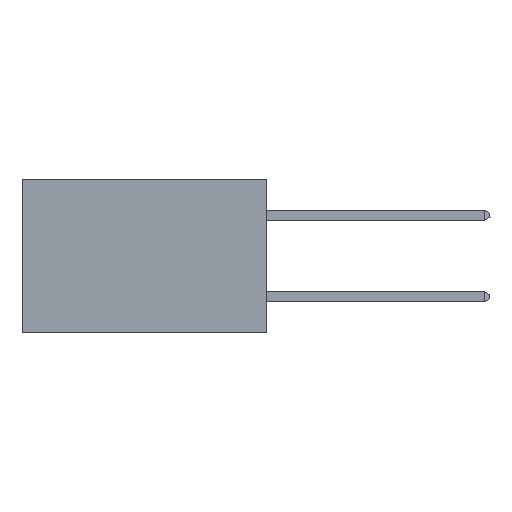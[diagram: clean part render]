
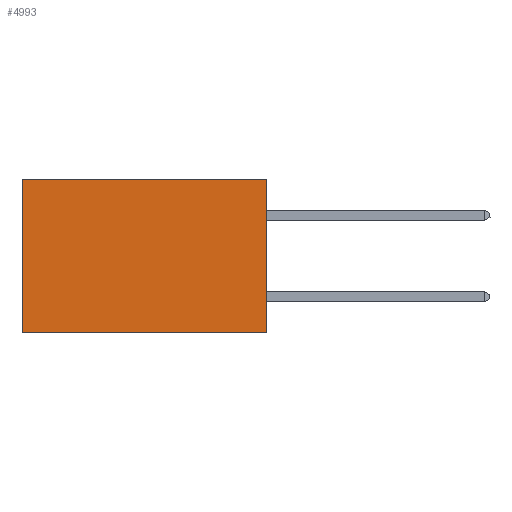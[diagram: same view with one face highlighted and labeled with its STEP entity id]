
A CAD part, left-side view. The second image highlights one B-rep face of the part: STEP entity #4993.
In plain terms, the highlighted planar face has unit normal (-1, 0, 0).
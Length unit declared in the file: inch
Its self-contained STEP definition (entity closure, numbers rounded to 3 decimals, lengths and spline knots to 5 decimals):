
#27 = DIRECTION ( 'NONE',  ( 0., 1., 0. ) ) ;
#249 = CARTESIAN_POINT ( 'NONE',  ( 0.2875, 0.6, -0.375 ) ) ;
#321 = VECTOR ( 'NONE', #4545, 39.37008 ) ;
#814 = VECTOR ( 'NONE', #3236, 39.37008 ) ;
#1058 = ORIENTED_EDGE ( 'NONE', *, *, #6612, .T. ) ;
#1090 = VERTEX_POINT ( 'NONE', #7222 ) ;
#1343 = VERTEX_POINT ( 'NONE', #3189 ) ;
#1454 = CARTESIAN_POINT ( 'NONE',  ( 0.2875, 0., -0.375 ) ) ;
#1946 = EDGE_CURVE ( 'NONE', #1343, #6137, #8209, .T. ) ;
#1982 = AXIS2_PLACEMENT_3D ( 'NONE', #2321, #8079, #8031 ) ;
#2321 = CARTESIAN_POINT ( 'NONE',  ( 0.2875, 0., -0.375 ) ) ;
#2535 = LINE ( 'NONE', #8260, #4358 ) ;
#2647 = EDGE_CURVE ( 'NONE', #6206, #1090, #6399, .T. ) ;
#2751 = LINE ( 'NONE', #6963, #321 ) ;
#3166 = ORIENTED_EDGE ( 'NONE', *, *, #1946, .F. ) ;
#3189 = CARTESIAN_POINT ( 'NONE',  ( 0.2875, 0., 0. ) ) ;
#3236 = DIRECTION ( 'NONE',  ( 0., 0., -1. ) ) ;
#4358 = VECTOR ( 'NONE', #27, 39.37008 ) ;
#4545 = DIRECTION ( 'NONE',  ( 0., 1., 0. ) ) ;
#4993 = ADVANCED_FACE ( 'NONE', ( #5554 ), #6759, .F. ) ;
#5202 = CARTESIAN_POINT ( 'NONE',  ( 0.2875, 0., -0.375 ) ) ;
#5303 = CARTESIAN_POINT ( 'NONE',  ( 0.2875, 0.6, 0. ) ) ;
#5501 = VECTOR ( 'NONE', #7814, 39.37008 ) ;
#5554 = FACE_OUTER_BOUND ( 'NONE', #6418, .T. ) ;
#5687 = ORIENTED_EDGE ( 'NONE', *, *, #2647, .T. ) ;
#6137 = VERTEX_POINT ( 'NONE', #1454 ) ;
#6206 = VERTEX_POINT ( 'NONE', #5303 ) ;
#6399 = LINE ( 'NONE', #249, #5501 ) ;
#6418 = EDGE_LOOP ( 'NONE', ( #5687, #6562, #3166, #1058 ) ) ;
#6562 = ORIENTED_EDGE ( 'NONE', *, *, #6587, .F. ) ;
#6587 = EDGE_CURVE ( 'NONE', #6137, #1090, #2751, .T. ) ;
#6612 = EDGE_CURVE ( 'NONE', #1343, #6206, #2535, .T. ) ;
#6759 = PLANE ( 'NONE',  #1982 ) ;
#6963 = CARTESIAN_POINT ( 'NONE',  ( 0.2875, 0., -0.375 ) ) ;
#7222 = CARTESIAN_POINT ( 'NONE',  ( 0.2875, 0.6, -0.375 ) ) ;
#7814 = DIRECTION ( 'NONE',  ( 0., 0., -1. ) ) ;
#8031 = DIRECTION ( 'NONE',  ( 0., 0., -1. ) ) ;
#8079 = DIRECTION ( 'NONE',  ( 1., 0., 0. ) ) ;
#8209 = LINE ( 'NONE', #5202, #814 ) ;
#8260 = CARTESIAN_POINT ( 'NONE',  ( 0.2875, 0., 0. ) ) ;
